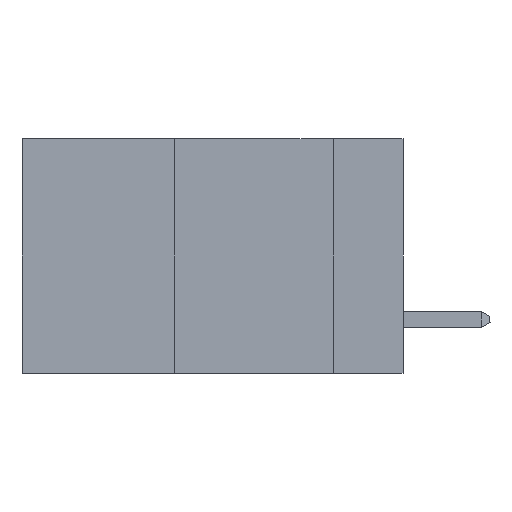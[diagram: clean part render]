
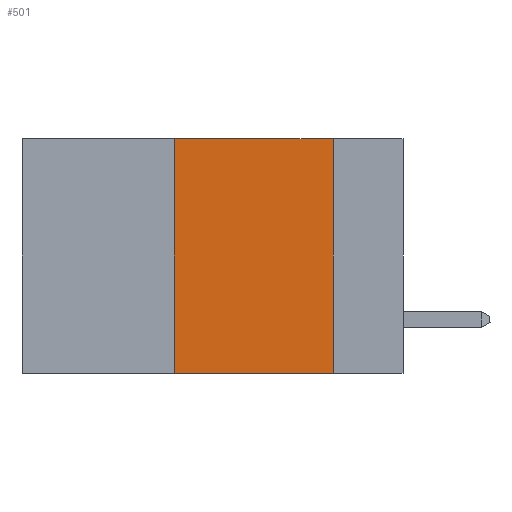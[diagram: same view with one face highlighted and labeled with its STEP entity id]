
A CAD part, left-side view. The second image highlights one B-rep face of the part: STEP entity #501.
In plain terms, the highlighted planar face has unit normal (-1, 0, 0).
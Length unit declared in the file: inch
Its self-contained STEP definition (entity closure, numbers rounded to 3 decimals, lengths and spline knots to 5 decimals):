
#501 = ADVANCED_FACE ( 'NONE', ( #1765 ), #11975, .F. ) ;
#849 = EDGE_CURVE ( 'NONE', #28331, #20844, #27039, .T. ) ;
#1126 = DIRECTION ( 'NONE',  ( 0., -1., 0. ) ) ;
#1765 = FACE_OUTER_BOUND ( 'NONE', #31190, .T. ) ;
#2472 = CARTESIAN_POINT ( 'NONE',  ( 0., 0.6, 0. ) ) ;
#2483 = VECTOR ( 'NONE', #11502, 39.37008 ) ;
#2673 = EDGE_CURVE ( 'NONE', #25865, #24056, #28508, .T. ) ;
#3153 = CARTESIAN_POINT ( 'NONE',  ( 0., 0.36, 0. ) ) ;
#4695 = DIRECTION ( 'NONE',  ( 0., -1., 0. ) ) ;
#5588 = EDGE_CURVE ( 'NONE', #20844, #24056, #30039, .T. ) ;
#6093 = VECTOR ( 'NONE', #1126, 39.37008 ) ;
#7394 = CARTESIAN_POINT ( 'NONE',  ( 0., 0.6, 0. ) ) ;
#9475 = DIRECTION ( 'NONE',  ( 0., 0., -1. ) ) ;
#11502 = DIRECTION ( 'NONE',  ( 0., 0., 1. ) ) ;
#11975 = PLANE ( 'NONE',  #21883 ) ;
#12144 = DIRECTION ( 'NONE',  ( 1., 0., 0. ) ) ;
#14842 = VECTOR ( 'NONE', #9475, 39.37008 ) ;
#16521 = ORIENTED_EDGE ( 'NONE', *, *, #849, .F. ) ;
#19025 = ORIENTED_EDGE ( 'NONE', *, *, #2673, .T. ) ;
#20010 = VECTOR ( 'NONE', #4695, 39.37008 ) ;
#20844 = VERTEX_POINT ( 'NONE', #26419 ) ;
#21773 = CARTESIAN_POINT ( 'NONE',  ( 0., 0.11, 0. ) ) ;
#21883 = AXIS2_PLACEMENT_3D ( 'NONE', #7394, #12144, #28263 ) ;
#22053 = CARTESIAN_POINT ( 'NONE',  ( 0., 0.6, -0.37 ) ) ;
#23337 = ORIENTED_EDGE ( 'NONE', *, *, #26298, .F. ) ;
#24056 = VERTEX_POINT ( 'NONE', #31174 ) ;
#25865 = VERTEX_POINT ( 'NONE', #35394 ) ;
#26298 = EDGE_CURVE ( 'NONE', #25865, #28331, #32682, .T. ) ;
#26419 = CARTESIAN_POINT ( 'NONE',  ( 0., 0.11, 0. ) ) ;
#27039 = LINE ( 'NONE', #2472, #6093 ) ;
#28263 = DIRECTION ( 'NONE',  ( 0., 0., -1. ) ) ;
#28331 = VERTEX_POINT ( 'NONE', #31991 ) ;
#28508 = LINE ( 'NONE', #22053, #20010 ) ;
#30039 = LINE ( 'NONE', #21773, #14842 ) ;
#31174 = CARTESIAN_POINT ( 'NONE',  ( 0., 0.11, -0.37 ) ) ;
#31190 = EDGE_LOOP ( 'NONE', ( #33145, #16521, #23337, #19025 ) ) ;
#31991 = CARTESIAN_POINT ( 'NONE',  ( 0., 0.36, 0. ) ) ;
#32682 = LINE ( 'NONE', #3153, #2483 ) ;
#33145 = ORIENTED_EDGE ( 'NONE', *, *, #5588, .F. ) ;
#35394 = CARTESIAN_POINT ( 'NONE',  ( 0., 0.36, -0.37 ) ) ;
